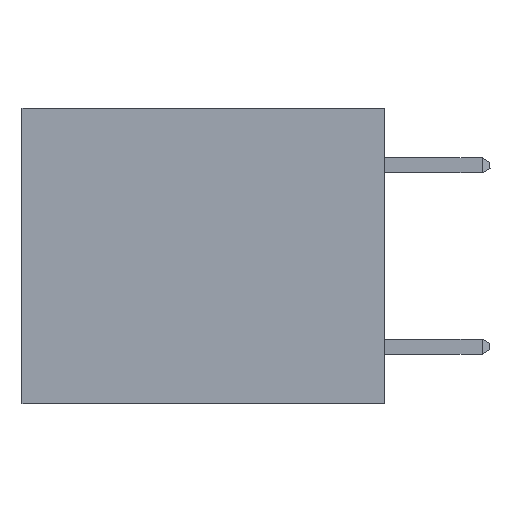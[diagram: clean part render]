
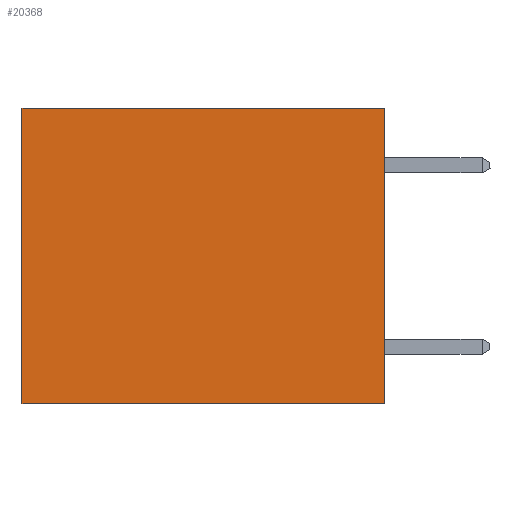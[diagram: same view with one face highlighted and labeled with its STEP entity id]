
A CAD part, left-side view. The second image highlights one B-rep face of the part: STEP entity #20368.
In plain terms, the highlighted planar face has unit normal (-1, 0, 0).
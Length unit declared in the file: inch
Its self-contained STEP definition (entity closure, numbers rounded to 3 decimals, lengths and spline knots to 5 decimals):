
#434 = ORIENTED_EDGE ( 'NONE', *, *, #4205, .F. ) ;
#533 = EDGE_CURVE ( 'NONE', #6180, #2094, #10570, .T. ) ;
#2094 = VERTEX_POINT ( 'NONE', #9981 ) ;
#2491 = CARTESIAN_POINT ( 'NONE',  ( 0.3165, 0.6, -0.49 ) ) ;
#2514 = LINE ( 'NONE', #2491, #2791 ) ;
#2566 = EDGE_CURVE ( 'NONE', #19641, #3345, #20742, .T. ) ;
#2791 = VECTOR ( 'NONE', #20444, 39.37008 ) ;
#3089 = LINE ( 'NONE', #5485, #17363 ) ;
#3345 = VERTEX_POINT ( 'NONE', #16706 ) ;
#4205 = EDGE_CURVE ( 'NONE', #6180, #19641, #3089, .T. ) ;
#4691 = PLANE ( 'NONE',  #17124 ) ;
#5485 = CARTESIAN_POINT ( 'NONE',  ( 0.3165, 0., -0.49 ) ) ;
#5847 = DIRECTION ( 'NONE',  ( 0., 0., -1. ) ) ;
#6180 = VERTEX_POINT ( 'NONE', #21820 ) ;
#6507 = VECTOR ( 'NONE', #21750, 39.37008 ) ;
#7469 = ORIENTED_EDGE ( 'NONE', *, *, #2566, .F. ) ;
#8620 = DIRECTION ( 'NONE',  ( 0., 0., -1. ) ) ;
#9069 = CARTESIAN_POINT ( 'NONE',  ( 0.3165, 0., -0.49 ) ) ;
#9981 = CARTESIAN_POINT ( 'NONE',  ( 0.3165, 0.6, 0. ) ) ;
#10181 = CARTESIAN_POINT ( 'NONE',  ( 0.3165, 0., -0.49 ) ) ;
#10570 = LINE ( 'NONE', #13595, #13626 ) ;
#13595 = CARTESIAN_POINT ( 'NONE',  ( 0.3165, 0., 0. ) ) ;
#13626 = VECTOR ( 'NONE', #18750, 39.37008 ) ;
#14516 = CARTESIAN_POINT ( 'NONE',  ( 0.3165, 0., -0.49 ) ) ;
#15909 = EDGE_CURVE ( 'NONE', #2094, #3345, #2514, .T. ) ;
#16706 = CARTESIAN_POINT ( 'NONE',  ( 0.3165, 0.6, -0.49 ) ) ;
#16897 = FACE_OUTER_BOUND ( 'NONE', #18596, .T. ) ;
#17124 = AXIS2_PLACEMENT_3D ( 'NONE', #10181, #19025, #8620 ) ;
#17225 = ORIENTED_EDGE ( 'NONE', *, *, #15909, .T. ) ;
#17363 = VECTOR ( 'NONE', #5847, 39.37008 ) ;
#18596 = EDGE_LOOP ( 'NONE', ( #17225, #7469, #434, #21521 ) ) ;
#18750 = DIRECTION ( 'NONE',  ( 0., 1., 0. ) ) ;
#19025 = DIRECTION ( 'NONE',  ( 1., 0., 0. ) ) ;
#19641 = VERTEX_POINT ( 'NONE', #9069 ) ;
#20368 = ADVANCED_FACE ( 'NONE', ( #16897 ), #4691, .F. ) ;
#20444 = DIRECTION ( 'NONE',  ( 0., 0., -1. ) ) ;
#20742 = LINE ( 'NONE', #14516, #6507 ) ;
#21521 = ORIENTED_EDGE ( 'NONE', *, *, #533, .T. ) ;
#21750 = DIRECTION ( 'NONE',  ( 0., 1., 0. ) ) ;
#21820 = CARTESIAN_POINT ( 'NONE',  ( 0.3165, 0., 0. ) ) ;
